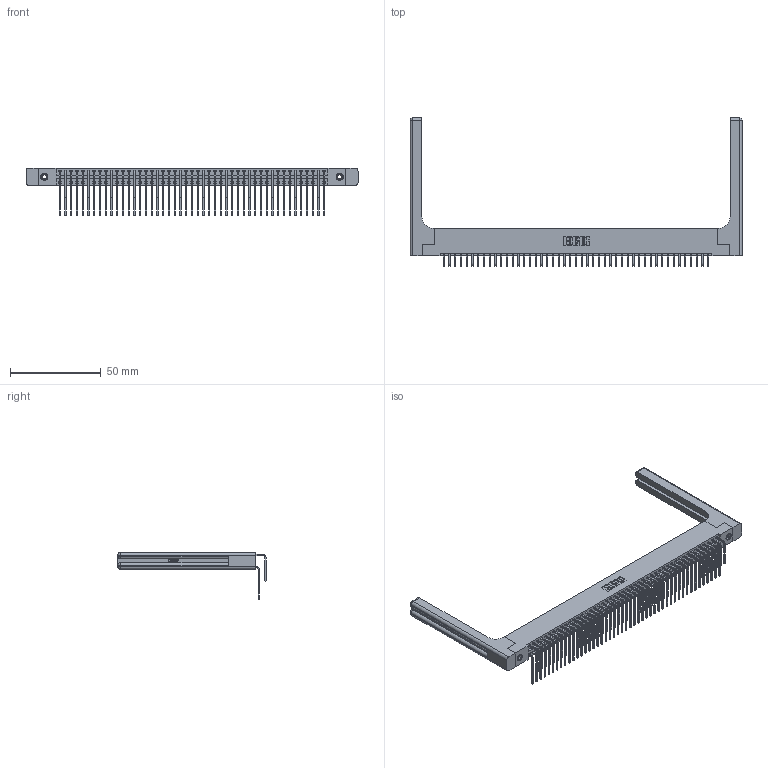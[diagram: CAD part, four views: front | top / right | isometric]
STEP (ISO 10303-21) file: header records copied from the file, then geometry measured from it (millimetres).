
FILE_DESCRIPTION (( 'STEP AP203' ), '1' );
FILE_NAME ('396-094-559-258.STEP', '2019-11-03T15:06:13', ( '' ), ( '' ), 'SwSTEP 2.0', 'SolidWorks 2016', '' );
FILE_SCHEMA (( 'CONFIG_CONTROL_DESIGN' ));
Length unit declared in the file: inch
Products named in the file (6): 346-220-058_345-220-058; 346 Part_Flush Mounting Lugs - 0.156 Dia-TH; 345-250-001_345-250-001-102; 345-292-001_558 559 Tail - 1; 396-094-559-258; 345-292-001_559 Tail - 2
Assembly tree (99 placements, depth 2):
  396-094-559-258
    346 Part_Flush Mounting Lugs - 0.156 Dia-TH
    345-292-001_558 559 Tail - 1  x47
    345-292-001_559 Tail - 2  x47
    345-250-001_345-250-001-102  x2
    346-220-058_345-220-058  x2
Bounding box: 183.29 x 81.85 x 26.16 mm (x, y, z)
Volume: 25948 mm3; surface area: 33018.8 mm2
Topology: 99 solids, 99 shells, 5454 faces, 16129 edges, 10606 vertices
Faces by surface type: plane 3702, cylinder 1692, bspline 36, cone 12, sphere 8, torus 4
Entity records: 36966 total; most frequent: CARTESIAN_POINT 7144, ORIENTED_EDGE 5824, DIRECTION 5252, EDGE_CURVE 2912, LINE 2460, VECTOR 2460, VERTEX_POINT 1930, AXIS2_PLACEMENT_3D 1396
